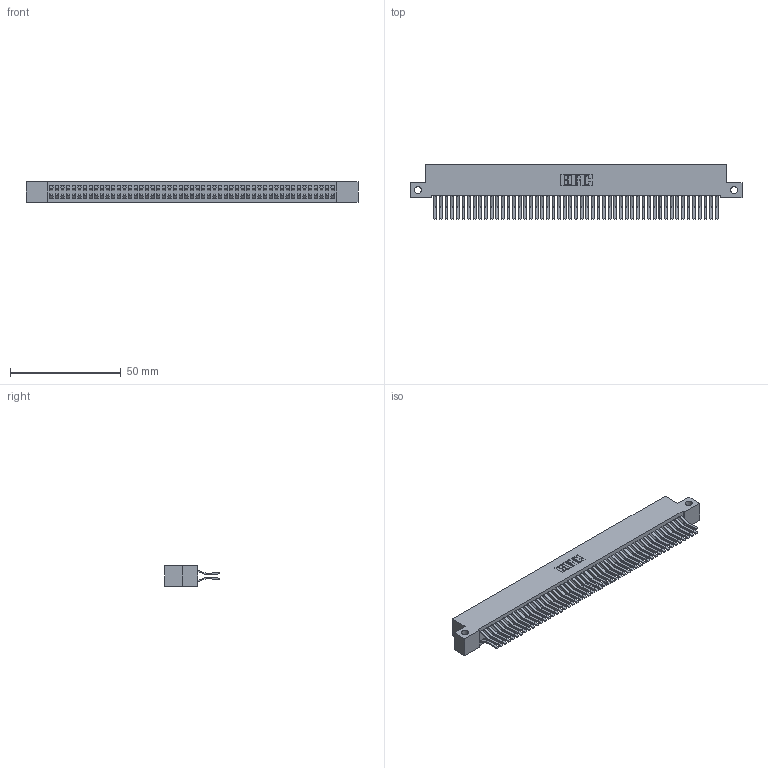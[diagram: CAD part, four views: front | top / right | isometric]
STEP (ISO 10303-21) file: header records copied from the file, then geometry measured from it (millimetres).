
FILE_DESCRIPTION (( 'STEP AP203' ), '1' );
FILE_NAME ('392-102-560-212.STEP', '2019-10-09T21:44:58', ( '' ), ( '' ), 'SwSTEP 2.0', 'SolidWorks 2016', '' );
FILE_SCHEMA (( 'CONFIG_CONTROL_DESIGN' ));
Length unit declared in the file: inch
Products named in the file (3): 342 Part_Side Mount; 345-292-001_560 Tail; 392-102-560-212
Assembly tree (103 placements, depth 2):
  392-102-560-212
    342 Part_Side Mount
    345-292-001_560 Tail  x102
Bounding box: 149.86 x 24.78 x 9.4 mm (x, y, z)
Volume: 14103.2 mm3; surface area: 24624.3 mm2
Topology: 103 solids, 103 shells, 5618 faces, 16721 edges, 11010 vertices
Faces by surface type: plane 3738, cylinder 1880
Entity records: 31605 total; most frequent: CARTESIAN_POINT 5226, ORIENTED_EDGE 5162, DIRECTION 4453, EDGE_CURVE 2581, LINE 2449, VECTOR 2449, VERTEX_POINT 1718, AXIS2_PLACEMENT_3D 1002
